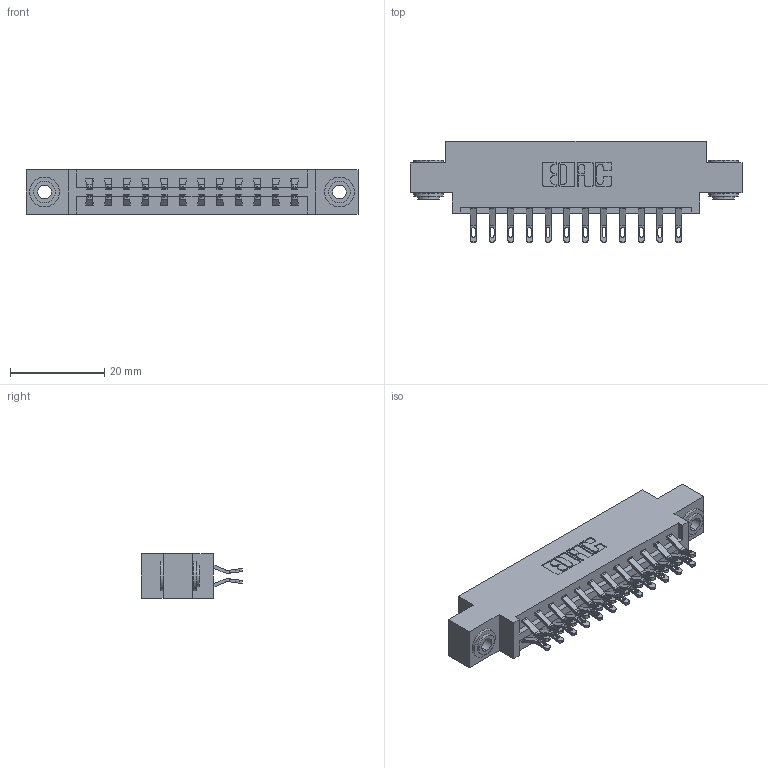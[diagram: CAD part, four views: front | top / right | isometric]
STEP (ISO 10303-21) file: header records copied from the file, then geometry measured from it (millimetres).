
FILE_DESCRIPTION (( 'STEP AP203' ), '1' );
FILE_NAME ('337-024-555-803.STEP', '2019-10-10T21:07:41', ( '' ), ( '' ), 'SwSTEP 2.0', 'SolidWorks 2016', '' );
FILE_SCHEMA (( 'CONFIG_CONTROL_DESIGN' ));
Length unit declared in the file: inch
Products named in the file (4): 345-250-002_345-250-002-102; 337 Part_0.170 Offset - 0.156 Dia-TH; 337-024-555-803; 345-292-001_555 Tail
Assembly tree (27 placements, depth 2):
  337-024-555-803
    337 Part_0.170 Offset - 0.156 Dia-TH
    345-292-001_555 Tail  x24
    345-250-002_345-250-002-102  x2
Bounding box: 70.56 x 21.47 x 9.4 mm (x, y, z)
Volume: 7008.5 mm3; surface area: 8226.3 mm2
Topology: 27 solids, 27 shells, 1596 faces, 4935 edges, 3286 vertices
Faces by surface type: plane 948, cylinder 640, cone 8
Entity records: 14292 total; most frequent: CARTESIAN_POINT 2443, ORIENTED_EDGE 2342, DIRECTION 2137, EDGE_CURVE 1171, LINE 999, VECTOR 999, VERTEX_POINT 778, AXIS2_PLACEMENT_3D 569
